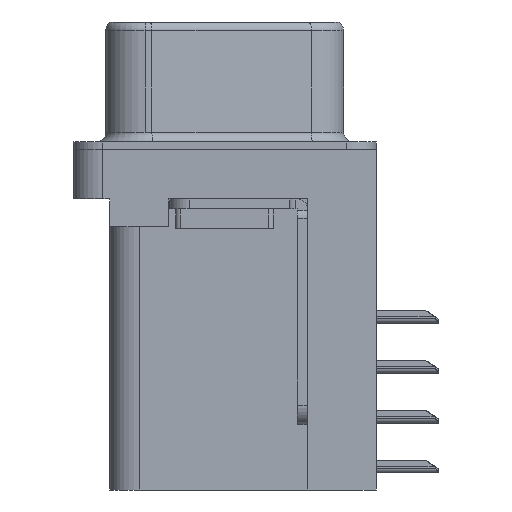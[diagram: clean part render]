
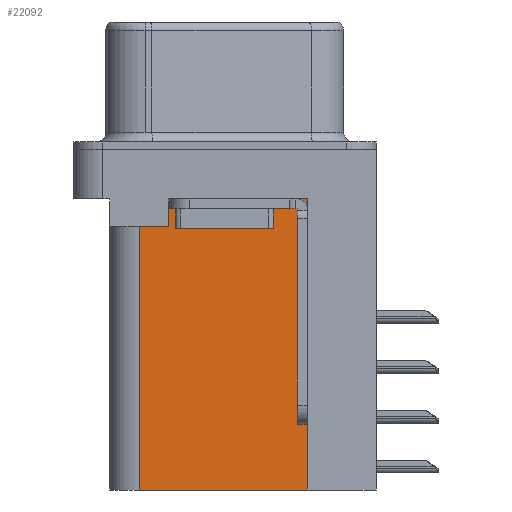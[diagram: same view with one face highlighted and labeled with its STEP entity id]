
A CAD part, left-side view. The second image highlights one B-rep face of the part: STEP entity #22092.
In plain terms, the highlighted planar face has unit normal (-1, 0, 0).
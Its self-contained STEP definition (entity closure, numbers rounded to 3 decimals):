
#447 = CARTESIAN_POINT ( 'NONE',  ( 3.75, 4.35, -17.3 ) ) ;
#965 = LINE ( 'NONE', #32570, #16679 ) ;
#2189 = DIRECTION ( 'NONE',  ( 1., 0., 0. ) ) ;
#2470 = CARTESIAN_POINT ( 'NONE',  ( 3.75, -4.2, -17.3 ) ) ;
#4953 = FACE_OUTER_BOUND ( 'NONE', #13529, .T. ) ;
#5949 = ORIENTED_EDGE ( 'NONE', *, *, #31071, .T. ) ;
#6370 = CARTESIAN_POINT ( 'NONE',  ( 3.75, -4.2, -17.3 ) ) ;
#6957 = CARTESIAN_POINT ( 'NONE',  ( 3.75, 2.85, -3.9 ) ) ;
#7160 = ORIENTED_EDGE ( 'NONE', *, *, #37741, .T. ) ;
#7215 = ORIENTED_EDGE ( 'NONE', *, *, #20647, .T. ) ;
#7758 = VECTOR ( 'NONE', #34384, 1000. ) ;
#9023 = CARTESIAN_POINT ( 'NONE',  ( 3.75, 4.35, -17.3 ) ) ;
#9696 = EDGE_CURVE ( 'NONE', #24483, #36354, #39786, .T. ) ;
#9714 = LINE ( 'NONE', #9023, #7758 ) ;
#9730 = CARTESIAN_POINT ( 'NONE',  ( 3.75, -4.2, -17.3 ) ) ;
#10572 = CARTESIAN_POINT ( 'NONE',  ( 3.75, 2.85, -3.9 ) ) ;
#11110 = EDGE_CURVE ( 'NONE', #36928, #28223, #40465, .T. ) ;
#13529 = EDGE_LOOP ( 'NONE', ( #7215, #25623, #7160, #26079, #37893, #5949 ) ) ;
#14572 = VERTEX_POINT ( 'NONE', #29155 ) ;
#16134 = CARTESIAN_POINT ( 'NONE',  ( 3.75, -4.2, -2.5 ) ) ;
#16679 = VECTOR ( 'NONE', #16737, 1000. ) ;
#16737 = DIRECTION ( 'NONE',  ( 0., 1., 0. ) ) ;
#18239 = CARTESIAN_POINT ( 'NONE',  ( 3.75, 4.35, -3.9 ) ) ;
#19827 = CARTESIAN_POINT ( 'NONE',  ( 3.75, 2.85, -2.5 ) ) ;
#20647 = EDGE_CURVE ( 'NONE', #14572, #24483, #30225, .T. ) ;
#21002 = CARTESIAN_POINT ( 'NONE',  ( 3.75, -4.2, -17.3 ) ) ;
#21294 = DIRECTION ( 'NONE',  ( 0., 0., 1. ) ) ;
#22092 = ADVANCED_FACE ( 'NONE', ( #4953 ), #36887, .F. ) ;
#22188 = VERTEX_POINT ( 'NONE', #18239 ) ;
#23811 = VECTOR ( 'NONE', #32744, 1000. ) ;
#24198 = DIRECTION ( 'NONE',  ( 0., 1., 0. ) ) ;
#24483 = VERTEX_POINT ( 'NONE', #19827 ) ;
#25623 = ORIENTED_EDGE ( 'NONE', *, *, #9696, .T. ) ;
#26079 = ORIENTED_EDGE ( 'NONE', *, *, #33278, .F. ) ;
#28223 = VERTEX_POINT ( 'NONE', #447 ) ;
#28244 = VECTOR ( 'NONE', #31965, 1000. ) ;
#29155 = CARTESIAN_POINT ( 'NONE',  ( 3.75, -4.2, -2.5 ) ) ;
#30225 = LINE ( 'NONE', #16134, #28244 ) ;
#30948 = VECTOR ( 'NONE', #38293, 1000. ) ;
#31071 = EDGE_CURVE ( 'NONE', #36928, #14572, #40655, .T. ) ;
#31221 = AXIS2_PLACEMENT_3D ( 'NONE', #21002, #2189, #24198 ) ;
#31965 = DIRECTION ( 'NONE',  ( 0., 1., 0. ) ) ;
#32158 = VECTOR ( 'NONE', #21294, 1000. ) ;
#32570 = CARTESIAN_POINT ( 'NONE',  ( 3.75, 0., -3.9 ) ) ;
#32744 = DIRECTION ( 'NONE',  ( 0., 0., -1. ) ) ;
#33278 = EDGE_CURVE ( 'NONE', #28223, #22188, #9714, .T. ) ;
#34384 = DIRECTION ( 'NONE',  ( 0., 0., 1. ) ) ;
#36354 = VERTEX_POINT ( 'NONE', #6957 ) ;
#36887 = PLANE ( 'NONE',  #31221 ) ;
#36928 = VERTEX_POINT ( 'NONE', #6370 ) ;
#37741 = EDGE_CURVE ( 'NONE', #36354, #22188, #965, .T. ) ;
#37893 = ORIENTED_EDGE ( 'NONE', *, *, #11110, .F. ) ;
#38293 = DIRECTION ( 'NONE',  ( 0., 1., 0. ) ) ;
#39786 = LINE ( 'NONE', #10572, #23811 ) ;
#40465 = LINE ( 'NONE', #9730, #30948 ) ;
#40655 = LINE ( 'NONE', #2470, #32158 ) ;
